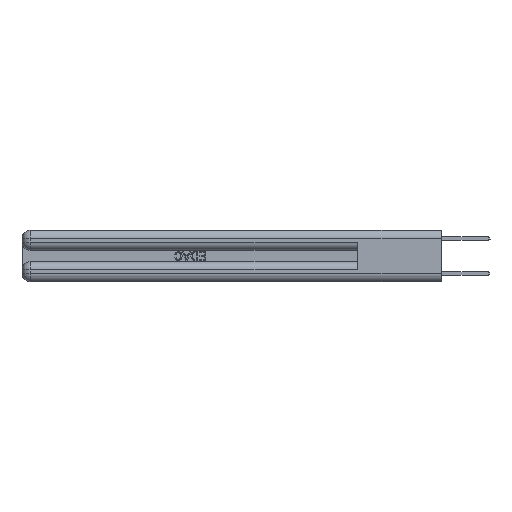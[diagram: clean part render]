
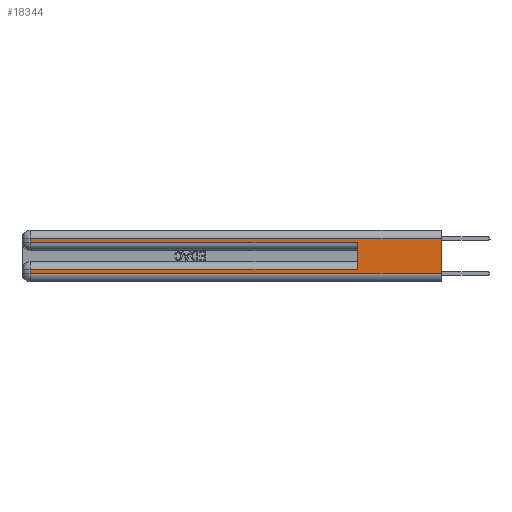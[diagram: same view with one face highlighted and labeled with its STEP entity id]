
A CAD part, left-side view. The second image highlights one B-rep face of the part: STEP entity #18344.
In plain terms, the highlighted planar face has unit normal (-1, 0, 0).
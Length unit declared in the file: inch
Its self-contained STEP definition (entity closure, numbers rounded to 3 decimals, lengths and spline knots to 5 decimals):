
#268 = CARTESIAN_POINT ( 'NONE',  ( 0., 0.6, 0.145 ) ) ;
#807 = DIRECTION ( 'NONE',  ( 0., 0., -1. ) ) ;
#1128 = AXIS2_PLACEMENT_3D ( 'NONE', #29712, #19435, #30433 ) ;
#2105 = VERTEX_POINT ( 'NONE', #32563 ) ;
#2641 = EDGE_CURVE ( 'NONE', #34571, #27613, #11049, .T. ) ;
#2987 = LINE ( 'NONE', #22124, #29848 ) ;
#3607 = LINE ( 'NONE', #14083, #13708 ) ;
#3689 = ORIENTED_EDGE ( 'NONE', *, *, #18193, .F. ) ;
#4287 = ORIENTED_EDGE ( 'NONE', *, *, #2641, .T. ) ;
#4582 = CARTESIAN_POINT ( 'NONE',  ( 0., 0.6, 0.085 ) ) ;
#4694 = LINE ( 'NONE', #32848, #5051 ) ;
#4989 = VERTEX_POINT ( 'NONE', #4582 ) ;
#5051 = VECTOR ( 'NONE', #24019, 39.37008 ) ;
#5696 = LINE ( 'NONE', #268, #27183 ) ;
#5749 = VECTOR ( 'NONE', #9898, 39.37008 ) ;
#5832 = EDGE_CURVE ( 'NONE', #2105, #30249, #4694, .T. ) ;
#7517 = CARTESIAN_POINT ( 'NONE',  ( 0., 0., 0.285 ) ) ;
#7972 = EDGE_CURVE ( 'NONE', #14573, #14934, #12926, .T. ) ;
#9898 = DIRECTION ( 'NONE',  ( 0., 0., -1. ) ) ;
#11049 = LINE ( 'NONE', #14599, #26485 ) ;
#12790 = CARTESIAN_POINT ( 'NONE',  ( 0., 0., 0.37 ) ) ;
#12926 = LINE ( 'NONE', #7517, #18309 ) ;
#13013 = EDGE_CURVE ( 'NONE', #4989, #34571, #3607, .T. ) ;
#13708 = VECTOR ( 'NONE', #20388, 39.37008 ) ;
#13784 = ORIENTED_EDGE ( 'NONE', *, *, #13013, .T. ) ;
#14083 = CARTESIAN_POINT ( 'NONE',  ( 0., 0., 0.085 ) ) ;
#14573 = VERTEX_POINT ( 'NONE', #31724 ) ;
#14599 = CARTESIAN_POINT ( 'NONE',  ( 0., 2.94, 0.37 ) ) ;
#14809 = EDGE_CURVE ( 'NONE', #30249, #14573, #2987, .T. ) ;
#14811 = ORIENTED_EDGE ( 'NONE', *, *, #7972, .T. ) ;
#14861 = CARTESIAN_POINT ( 'NONE',  ( 0., 2.94, 0.31 ) ) ;
#14934 = VERTEX_POINT ( 'NONE', #34386 ) ;
#14993 = CARTESIAN_POINT ( 'NONE',  ( 0., 0., 0.06 ) ) ;
#15293 = LINE ( 'NONE', #12790, #5749 ) ;
#15304 = VERTEX_POINT ( 'NONE', #20936 ) ;
#16649 = ORIENTED_EDGE ( 'NONE', *, *, #14809, .T. ) ;
#16714 = CARTESIAN_POINT ( 'NONE',  ( 0., 2.94, 0.085 ) ) ;
#18193 = EDGE_CURVE ( 'NONE', #2105, #15304, #15293, .T. ) ;
#18309 = VECTOR ( 'NONE', #23768, 39.37008 ) ;
#18344 = ADVANCED_FACE ( 'NONE', ( #24486 ), #35491, .F. ) ;
#19435 = DIRECTION ( 'NONE',  ( 1., 0., 0. ) ) ;
#20388 = DIRECTION ( 'NONE',  ( 0., 1., 0. ) ) ;
#20936 = CARTESIAN_POINT ( 'NONE',  ( 0., 0., 0.06 ) ) ;
#21981 = EDGE_LOOP ( 'NONE', ( #3689, #29969, #16649, #14811, #33080, #13784, #4287, #25814 ) ) ;
#22124 = CARTESIAN_POINT ( 'NONE',  ( 0., 2.94, 0.37 ) ) ;
#23768 = DIRECTION ( 'NONE',  ( 0., -1., 0. ) ) ;
#24019 = DIRECTION ( 'NONE',  ( 0., 1., 0. ) ) ;
#24486 = FACE_OUTER_BOUND ( 'NONE', #21981, .T. ) ;
#25192 = DIRECTION ( 'NONE',  ( 0., 0., 1. ) ) ;
#25814 = ORIENTED_EDGE ( 'NONE', *, *, #28845, .T. ) ;
#26485 = VECTOR ( 'NONE', #28487, 39.37008 ) ;
#27183 = VECTOR ( 'NONE', #25192, 39.37008 ) ;
#27613 = VERTEX_POINT ( 'NONE', #34844 ) ;
#28487 = DIRECTION ( 'NONE',  ( 0., 0., -1. ) ) ;
#28845 = EDGE_CURVE ( 'NONE', #27613, #15304, #34295, .T. ) ;
#29255 = VECTOR ( 'NONE', #34485, 39.37008 ) ;
#29712 = CARTESIAN_POINT ( 'NONE',  ( 0., 0., 0.37 ) ) ;
#29848 = VECTOR ( 'NONE', #807, 39.37008 ) ;
#29969 = ORIENTED_EDGE ( 'NONE', *, *, #5832, .T. ) ;
#30249 = VERTEX_POINT ( 'NONE', #14861 ) ;
#30433 = DIRECTION ( 'NONE',  ( 0., 0., -1. ) ) ;
#31724 = CARTESIAN_POINT ( 'NONE',  ( 0., 2.94, 0.285 ) ) ;
#32563 = CARTESIAN_POINT ( 'NONE',  ( 0., 0., 0.31 ) ) ;
#32848 = CARTESIAN_POINT ( 'NONE',  ( 0., 0., 0.31 ) ) ;
#33080 = ORIENTED_EDGE ( 'NONE', *, *, #33580, .F. ) ;
#33580 = EDGE_CURVE ( 'NONE', #4989, #14934, #5696, .T. ) ;
#34295 = LINE ( 'NONE', #14993, #29255 ) ;
#34386 = CARTESIAN_POINT ( 'NONE',  ( 0., 0.6, 0.285 ) ) ;
#34485 = DIRECTION ( 'NONE',  ( 0., -1., 0. ) ) ;
#34571 = VERTEX_POINT ( 'NONE', #16714 ) ;
#34844 = CARTESIAN_POINT ( 'NONE',  ( 0., 2.94, 0.06 ) ) ;
#35491 = PLANE ( 'NONE',  #1128 ) ;
